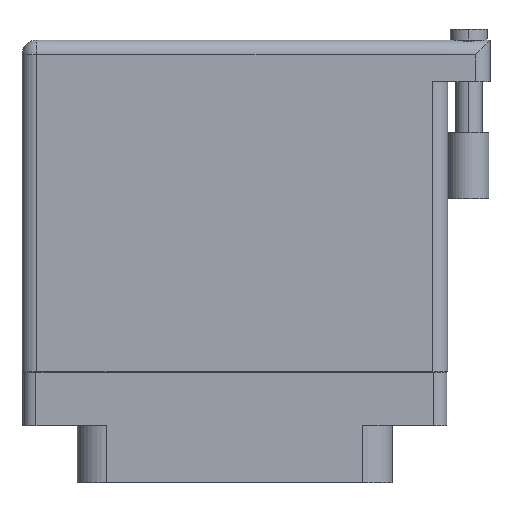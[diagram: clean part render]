
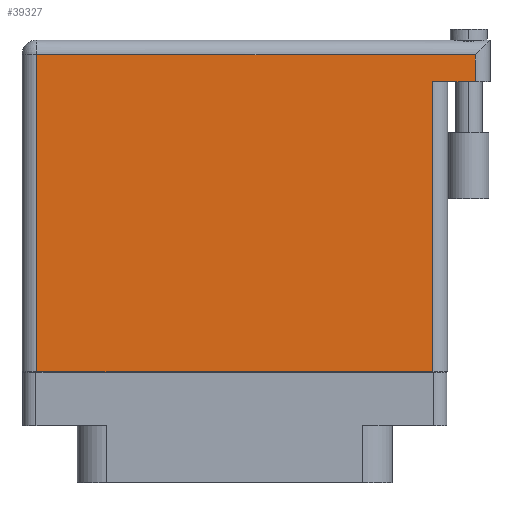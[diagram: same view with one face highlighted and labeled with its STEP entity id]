
A CAD part, front view. The second image highlights one B-rep face of the part: STEP entity #39327.
In plain terms, the highlighted face is planar.
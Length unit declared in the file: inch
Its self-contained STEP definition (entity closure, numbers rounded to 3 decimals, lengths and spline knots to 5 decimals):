
#172 = CARTESIAN_POINT ( 'NONE',  ( 0.934, 1.269, 0.4495 ) ) ;
#1652 = DIRECTION ( 'NONE',  ( 1., 0., 0. ) ) ;
#2176 = EDGE_CURVE ( 'NONE', #18258, #18686, #7468, .T. ) ;
#2939 = LINE ( 'NONE', #38276, #26432 ) ;
#4010 = ORIENTED_EDGE ( 'NONE', *, *, #19491, .T. ) ;
#4098 = DIRECTION ( 'NONE',  ( 0., 1., 0. ) ) ;
#4862 = LINE ( 'NONE', #37464, #25054 ) ;
#5334 = AXIS2_PLACEMENT_3D ( 'NONE', #17431, #17307, #20397 ) ;
#6400 = FACE_OUTER_BOUND ( 'NONE', #29081, .T. ) ;
#7468 = LINE ( 'NONE', #16935, #10857 ) ;
#8413 = ORIENTED_EDGE ( 'NONE', *, *, #10995, .T. ) ;
#10857 = VECTOR ( 'NONE', #1652, 39.37008 ) ;
#10995 = EDGE_CURVE ( 'NONE', #39740, #18258, #4862, .T. ) ;
#11003 = DIRECTION ( 'NONE',  ( -1., 0., 0. ) ) ;
#11830 = VERTEX_POINT ( 'NONE', #29879 ) ;
#16100 = CARTESIAN_POINT ( 'NONE',  ( 1.134, 1.466, 0.4495 ) ) ;
#16935 = CARTESIAN_POINT ( 'NONE',  ( -1.004, -0.1, 0.4495 ) ) ;
#16993 = EDGE_CURVE ( 'NONE', #11830, #29293, #2939, .T. ) ;
#17307 = DIRECTION ( 'NONE',  ( 0., 0., -1. ) ) ;
#17431 = CARTESIAN_POINT ( 'NONE',  ( -1.004, 1.466, 0.4495 ) ) ;
#17785 = ORIENTED_EDGE ( 'NONE', *, *, #16993, .F. ) ;
#18258 = VERTEX_POINT ( 'NONE', #28185 ) ;
#18686 = VERTEX_POINT ( 'NONE', #28264 ) ;
#19491 = EDGE_CURVE ( 'NONE', #11830, #33582, #29094, .T. ) ;
#19545 = VECTOR ( 'NONE', #21654, 39.37008 ) ;
#20397 = DIRECTION ( 'NONE',  ( -1., 0., 0. ) ) ;
#20972 = CARTESIAN_POINT ( 'NONE',  ( 1.134, 1.396, 0.4495 ) ) ;
#21202 = ORIENTED_EDGE ( 'NONE', *, *, #21992, .T. ) ;
#21654 = DIRECTION ( 'NONE',  ( 0., 1., 0. ) ) ;
#21992 = EDGE_CURVE ( 'NONE', #33582, #39740, #33701, .T. ) ;
#22614 = CARTESIAN_POINT ( 'NONE',  ( 0.934, 1.269, 0.4495 ) ) ;
#25029 = VECTOR ( 'NONE', #36362, 39.37008 ) ;
#25054 = VECTOR ( 'NONE', #35161, 39.37008 ) ;
#26188 = ORIENTED_EDGE ( 'NONE', *, *, #31314, .T. ) ;
#26432 = VECTOR ( 'NONE', #11003, 39.37008 ) ;
#28185 = CARTESIAN_POINT ( 'NONE',  ( -0.934, -0.1, 0.4495 ) ) ;
#28221 = ORIENTED_EDGE ( 'NONE', *, *, #2176, .T. ) ;
#28264 = CARTESIAN_POINT ( 'NONE',  ( 0.934, -0.1, 0.4495 ) ) ;
#28454 = CARTESIAN_POINT ( 'NONE',  ( -0.934, 1.396, 0.4495 ) ) ;
#29081 = EDGE_LOOP ( 'NONE', ( #28221, #26188, #17785, #4010, #21202, #8413 ) ) ;
#29094 = LINE ( 'NONE', #16100, #35318 ) ;
#29293 = VERTEX_POINT ( 'NONE', #22614 ) ;
#29879 = CARTESIAN_POINT ( 'NONE',  ( 1.134, 1.269, 0.4495 ) ) ;
#31314 = EDGE_CURVE ( 'NONE', #18686, #29293, #36331, .T. ) ;
#32895 = CARTESIAN_POINT ( 'NONE',  ( -1.004, 1.396, 0.4495 ) ) ;
#33582 = VERTEX_POINT ( 'NONE', #20972 ) ;
#33701 = LINE ( 'NONE', #32895, #25029 ) ;
#35161 = DIRECTION ( 'NONE',  ( 0., -1., 0. ) ) ;
#35318 = VECTOR ( 'NONE', #4098, 39.37008 ) ;
#35567 = PLANE ( 'NONE',  #5334 ) ;
#36331 = LINE ( 'NONE', #172, #19545 ) ;
#36362 = DIRECTION ( 'NONE',  ( -1., 0., 0. ) ) ;
#37464 = CARTESIAN_POINT ( 'NONE',  ( -0.934, -0.1, 0.4495 ) ) ;
#38276 = CARTESIAN_POINT ( 'NONE',  ( 1.204, 1.269, 0.4495 ) ) ;
#39327 = ADVANCED_FACE ( 'NONE', ( #6400 ), #35567, .F. ) ;
#39740 = VERTEX_POINT ( 'NONE', #28454 ) ;
